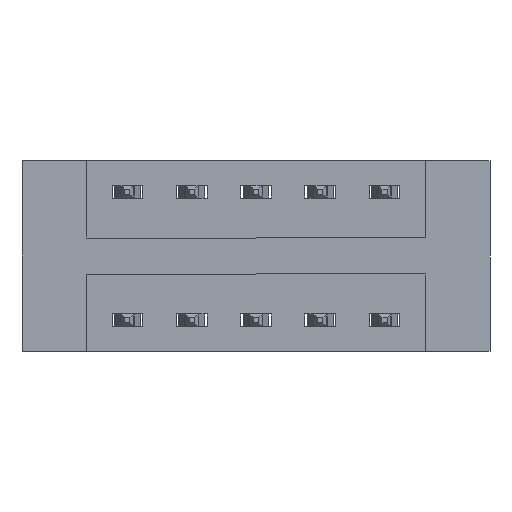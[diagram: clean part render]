
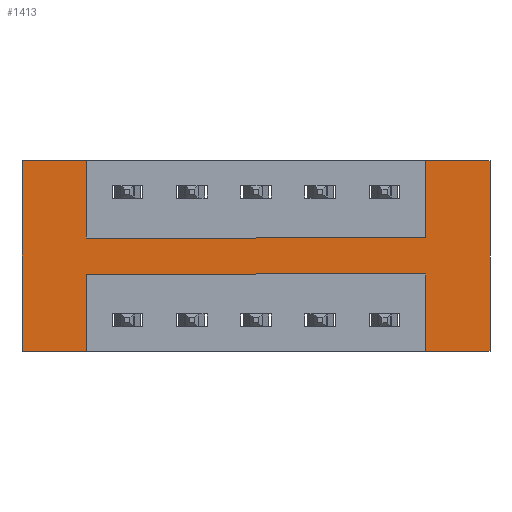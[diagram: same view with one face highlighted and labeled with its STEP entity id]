
A CAD part, front view. The second image highlights one B-rep face of the part: STEP entity #1413.
In plain terms, the highlighted planar face has unit normal (0, -1, 0).
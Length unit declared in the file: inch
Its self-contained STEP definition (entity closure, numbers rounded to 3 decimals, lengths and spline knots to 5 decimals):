
#34 = CARTESIAN_POINT ( 'NONE',  ( 0., 0., -0.37 ) ) ;
#50 = VERTEX_POINT ( 'NONE', #7156 ) ;
#208 = VERTEX_POINT ( 'NONE', #5497 ) ;
#249 = EDGE_CURVE ( 'NONE', #5957, #208, #5055, .T. ) ;
#271 = CARTESIAN_POINT ( 'NONE',  ( 1.0475, 0., -0.37 ) ) ;
#272 = VERTEX_POINT ( 'NONE', #1602 ) ;
#309 = DIRECTION ( 'NONE',  ( 0., 0., -1. ) ) ;
#396 = DIRECTION ( 'NONE',  ( 1., 0., 0. ) ) ;
#584 = ORIENTED_EDGE ( 'NONE', *, *, #3803, .F. ) ;
#612 = CARTESIAN_POINT ( 'NONE',  ( 0., 0., 0. ) ) ;
#801 = EDGE_CURVE ( 'NONE', #4224, #6697, #1554, .T. ) ;
#808 = VERTEX_POINT ( 'NONE', #2667 ) ;
#968 = CARTESIAN_POINT ( 'NONE',  ( 1.0475, 0., -0.22 ) ) ;
#1327 = VECTOR ( 'NONE', #2460, 39.37008 ) ;
#1338 = DIRECTION ( 'NONE',  ( 1., 0., 0. ) ) ;
#1413 = ADVANCED_FACE ( 'NONE', ( #6480 ), #7086, .T. ) ;
#1554 = LINE ( 'NONE', #2789, #3235 ) ;
#1602 = CARTESIAN_POINT ( 'NONE',  ( 0.3875, 0., -0.15 ) ) ;
#1624 = CARTESIAN_POINT ( 'NONE',  ( 0.2625, 0., 0. ) ) ;
#1632 = LINE ( 'NONE', #7487, #6319 ) ;
#1647 = CARTESIAN_POINT ( 'NONE',  ( 0., 0., -0.37 ) ) ;
#1663 = DIRECTION ( 'NONE',  ( 0., 0., -1. ) ) ;
#1883 = VECTOR ( 'NONE', #7710, 39.37008 ) ;
#2173 = VECTOR ( 'NONE', #309, 39.37008 ) ;
#2272 = ORIENTED_EDGE ( 'NONE', *, *, #4733, .F. ) ;
#2378 = ORIENTED_EDGE ( 'NONE', *, *, #7965, .F. ) ;
#2428 = VECTOR ( 'NONE', #1338, 39.37008 ) ;
#2460 = DIRECTION ( 'NONE',  ( 0., 0., 1. ) ) ;
#2483 = ORIENTED_EDGE ( 'NONE', *, *, #3011, .F. ) ;
#2663 = ORIENTED_EDGE ( 'NONE', *, *, #7801, .F. ) ;
#2667 = CARTESIAN_POINT ( 'NONE',  ( 0.3875, 0., 0. ) ) ;
#2789 = CARTESIAN_POINT ( 'NONE',  ( 1.1725, 0., 0. ) ) ;
#2793 = DIRECTION ( 'NONE',  ( -1., 0., 0. ) ) ;
#2814 = DIRECTION ( 'NONE',  ( 0., 0., 1. ) ) ;
#2858 = DIRECTION ( 'NONE',  ( 1., 0., 0. ) ) ;
#2865 = ORIENTED_EDGE ( 'NONE', *, *, #3509, .F. ) ;
#2917 = CARTESIAN_POINT ( 'NONE',  ( 1.0475, 0., -0.37 ) ) ;
#3011 = EDGE_CURVE ( 'NONE', #272, #50, #3444, .T. ) ;
#3105 = VERTEX_POINT ( 'NONE', #6167 ) ;
#3156 = EDGE_LOOP ( 'NONE', ( #6910, #2272, #3929, #2483, #4133, #2663, #5911, #2865, #4706, #3842, #584, #2378 ) ) ;
#3235 = VECTOR ( 'NONE', #2814, 39.37008 ) ;
#3343 = CARTESIAN_POINT ( 'NONE',  ( 0.3875, 0., -0.37 ) ) ;
#3412 = VERTEX_POINT ( 'NONE', #3343 ) ;
#3430 = VECTOR ( 'NONE', #5834, 39.37008 ) ;
#3444 = LINE ( 'NONE', #4319, #6281 ) ;
#3477 = CARTESIAN_POINT ( 'NONE',  ( 0., 0., 0. ) ) ;
#3509 = EDGE_CURVE ( 'NONE', #3412, #208, #3648, .T. ) ;
#3538 = LINE ( 'NONE', #271, #1883 ) ;
#3539 = LINE ( 'NONE', #3477, #6366 ) ;
#3648 = LINE ( 'NONE', #34, #5065 ) ;
#3803 = EDGE_CURVE ( 'NONE', #6506, #6524, #3538, .T. ) ;
#3842 = ORIENTED_EDGE ( 'NONE', *, *, #5513, .F. ) ;
#3929 = ORIENTED_EDGE ( 'NONE', *, *, #6735, .F. ) ;
#4133 = ORIENTED_EDGE ( 'NONE', *, *, #6877, .F. ) ;
#4171 = DIRECTION ( 'NONE',  ( 0., 0., -1. ) ) ;
#4224 = VERTEX_POINT ( 'NONE', #6643 ) ;
#4319 = CARTESIAN_POINT ( 'NONE',  ( 0.3875, 0., -0.15 ) ) ;
#4706 = ORIENTED_EDGE ( 'NONE', *, *, #4923, .F. ) ;
#4733 = EDGE_CURVE ( 'NONE', #3105, #6697, #3539, .T. ) ;
#4923 = EDGE_CURVE ( 'NONE', #6578, #3412, #5637, .T. ) ;
#5053 = LINE ( 'NONE', #7491, #3430 ) ;
#5055 = LINE ( 'NONE', #1624, #5439 ) ;
#5065 = VECTOR ( 'NONE', #6430, 39.37008 ) ;
#5233 = AXIS2_PLACEMENT_3D ( 'NONE', #1647, #7609, #4171 ) ;
#5313 = LINE ( 'NONE', #7836, #5517 ) ;
#5439 = VECTOR ( 'NONE', #1663, 39.37008 ) ;
#5464 = CARTESIAN_POINT ( 'NONE',  ( 1.1725, 0., 0. ) ) ;
#5497 = CARTESIAN_POINT ( 'NONE',  ( 0.2625, 0., -0.37 ) ) ;
#5513 = EDGE_CURVE ( 'NONE', #6524, #6578, #5053, .T. ) ;
#5517 = VECTOR ( 'NONE', #5623, 39.37008 ) ;
#5623 = DIRECTION ( 'NONE',  ( 0., 0., -1. ) ) ;
#5637 = LINE ( 'NONE', #6610, #2173 ) ;
#5834 = DIRECTION ( 'NONE',  ( -1., 0., 0. ) ) ;
#5911 = ORIENTED_EDGE ( 'NONE', *, *, #249, .T. ) ;
#5957 = VERTEX_POINT ( 'NONE', #6174 ) ;
#6167 = CARTESIAN_POINT ( 'NONE',  ( 1.0475, 0., 0. ) ) ;
#6174 = CARTESIAN_POINT ( 'NONE',  ( 0.2625, 0., 0. ) ) ;
#6250 = LINE ( 'NONE', #6696, #1327 ) ;
#6281 = VECTOR ( 'NONE', #396, 39.37008 ) ;
#6319 = VECTOR ( 'NONE', #2793, 39.37008 ) ;
#6366 = VECTOR ( 'NONE', #2858, 39.37008 ) ;
#6430 = DIRECTION ( 'NONE',  ( -1., 0., 0. ) ) ;
#6480 = FACE_OUTER_BOUND ( 'NONE', #3156, .T. ) ;
#6506 = VERTEX_POINT ( 'NONE', #2917 ) ;
#6524 = VERTEX_POINT ( 'NONE', #968 ) ;
#6578 = VERTEX_POINT ( 'NONE', #6590 ) ;
#6590 = CARTESIAN_POINT ( 'NONE',  ( 0.3875, 0., -0.22 ) ) ;
#6610 = CARTESIAN_POINT ( 'NONE',  ( 0.3875, 0., -0.37 ) ) ;
#6643 = CARTESIAN_POINT ( 'NONE',  ( 1.1725, 0., -0.37 ) ) ;
#6696 = CARTESIAN_POINT ( 'NONE',  ( 1.0475, 0., 0. ) ) ;
#6697 = VERTEX_POINT ( 'NONE', #5464 ) ;
#6735 = EDGE_CURVE ( 'NONE', #50, #3105, #6250, .T. ) ;
#6877 = EDGE_CURVE ( 'NONE', #808, #272, #5313, .T. ) ;
#6910 = ORIENTED_EDGE ( 'NONE', *, *, #801, .T. ) ;
#7086 = PLANE ( 'NONE',  #5233 ) ;
#7156 = CARTESIAN_POINT ( 'NONE',  ( 1.0475, 0., -0.15 ) ) ;
#7194 = LINE ( 'NONE', #612, #2428 ) ;
#7487 = CARTESIAN_POINT ( 'NONE',  ( 0., 0., -0.37 ) ) ;
#7491 = CARTESIAN_POINT ( 'NONE',  ( 0.3875, 0., -0.22 ) ) ;
#7609 = DIRECTION ( 'NONE',  ( 0., -1., 0. ) ) ;
#7710 = DIRECTION ( 'NONE',  ( 0., 0., 1. ) ) ;
#7801 = EDGE_CURVE ( 'NONE', #5957, #808, #7194, .T. ) ;
#7836 = CARTESIAN_POINT ( 'NONE',  ( 0.3875, 0., 0. ) ) ;
#7965 = EDGE_CURVE ( 'NONE', #4224, #6506, #1632, .T. ) ;
